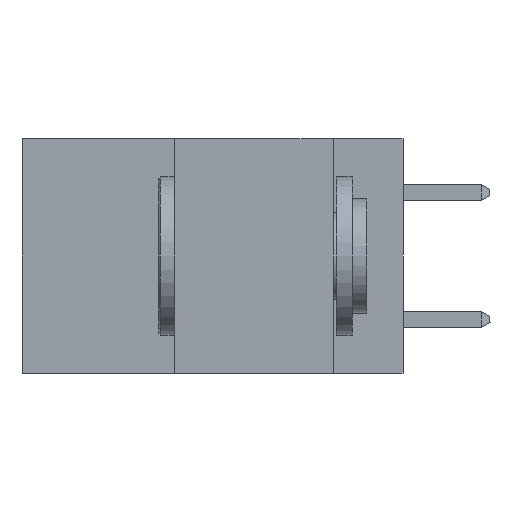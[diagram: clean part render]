
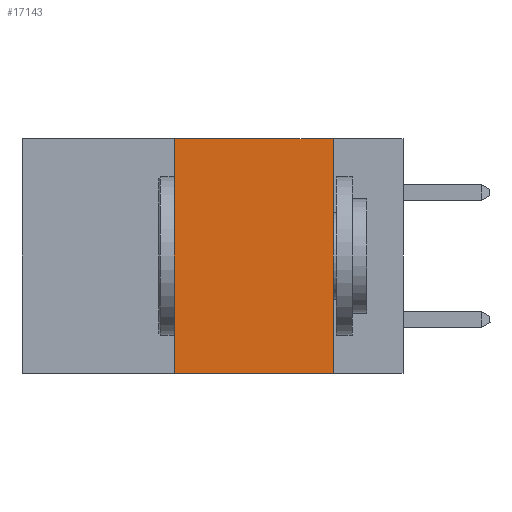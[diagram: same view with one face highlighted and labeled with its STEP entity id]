
A CAD part, left-side view. The second image highlights one B-rep face of the part: STEP entity #17143.
In plain terms, the highlighted planar face has unit normal (-1, 0, 0).
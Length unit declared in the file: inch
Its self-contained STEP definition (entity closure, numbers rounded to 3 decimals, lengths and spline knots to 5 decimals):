
#1400 = EDGE_CURVE ( 'NONE', #20414, #9456, #11640, .T. ) ;
#2141 = DIRECTION ( 'NONE',  ( 0., 0., 1. ) ) ;
#2501 = AXIS2_PLACEMENT_3D ( 'NONE', #17108, #6538, #18835 ) ;
#2538 = VECTOR ( 'NONE', #22635, 39.37008 ) ;
#4071 = CARTESIAN_POINT ( 'NONE',  ( 0., 0.36, 0. ) ) ;
#4701 = LINE ( 'NONE', #17610, #5280 ) ;
#4702 = PLANE ( 'NONE',  #2501 ) ;
#4790 = LINE ( 'NONE', #12188, #14805 ) ;
#5006 = ORIENTED_EDGE ( 'NONE', *, *, #1400, .T. ) ;
#5280 = VECTOR ( 'NONE', #22784, 39.37008 ) ;
#6538 = DIRECTION ( 'NONE',  ( 1., 0., 0. ) ) ;
#7198 = EDGE_CURVE ( 'NONE', #19461, #9456, #4701, .T. ) ;
#7828 = ORIENTED_EDGE ( 'NONE', *, *, #11154, .F. ) ;
#8594 = EDGE_LOOP ( 'NONE', ( #16067, #7828, #21563, #5006 ) ) ;
#9456 = VERTEX_POINT ( 'NONE', #11434 ) ;
#10100 = EDGE_CURVE ( 'NONE', #20414, #15481, #13558, .T. ) ;
#10252 = CARTESIAN_POINT ( 'NONE',  ( 0., 0.11, 0. ) ) ;
#11154 = EDGE_CURVE ( 'NONE', #15481, #19461, #4790, .T. ) ;
#11430 = CARTESIAN_POINT ( 'NONE',  ( 0., 0.36, -0.37 ) ) ;
#11434 = CARTESIAN_POINT ( 'NONE',  ( 0., 0.11, -0.37 ) ) ;
#11640 = LINE ( 'NONE', #13671, #2538 ) ;
#12188 = CARTESIAN_POINT ( 'NONE',  ( 0., 0.6, 0. ) ) ;
#13558 = LINE ( 'NONE', #4071, #22248 ) ;
#13671 = CARTESIAN_POINT ( 'NONE',  ( 0., 0.6, -0.37 ) ) ;
#13949 = DIRECTION ( 'NONE',  ( 0., -1., 0. ) ) ;
#14172 = FACE_OUTER_BOUND ( 'NONE', #8594, .T. ) ;
#14805 = VECTOR ( 'NONE', #13949, 39.37008 ) ;
#15481 = VERTEX_POINT ( 'NONE', #16296 ) ;
#16067 = ORIENTED_EDGE ( 'NONE', *, *, #7198, .F. ) ;
#16296 = CARTESIAN_POINT ( 'NONE',  ( 0., 0.36, 0. ) ) ;
#17108 = CARTESIAN_POINT ( 'NONE',  ( 0., 0.6, 0. ) ) ;
#17143 = ADVANCED_FACE ( 'NONE', ( #14172 ), #4702, .F. ) ;
#17610 = CARTESIAN_POINT ( 'NONE',  ( 0., 0.11, 0. ) ) ;
#18835 = DIRECTION ( 'NONE',  ( 0., 0., -1. ) ) ;
#19461 = VERTEX_POINT ( 'NONE', #10252 ) ;
#20414 = VERTEX_POINT ( 'NONE', #11430 ) ;
#21563 = ORIENTED_EDGE ( 'NONE', *, *, #10100, .F. ) ;
#22248 = VECTOR ( 'NONE', #2141, 39.37008 ) ;
#22635 = DIRECTION ( 'NONE',  ( 0., -1., 0. ) ) ;
#22784 = DIRECTION ( 'NONE',  ( 0., 0., -1. ) ) ;
